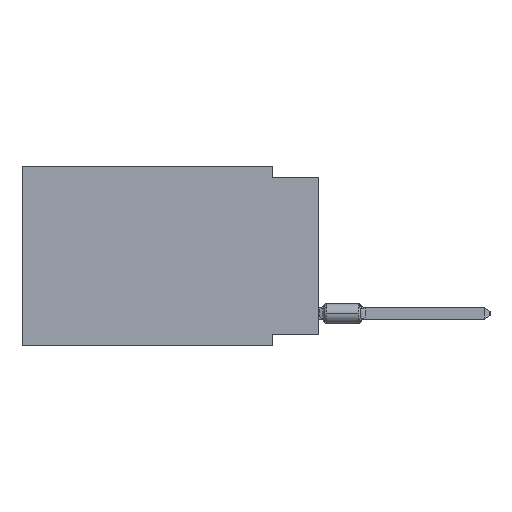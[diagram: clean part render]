
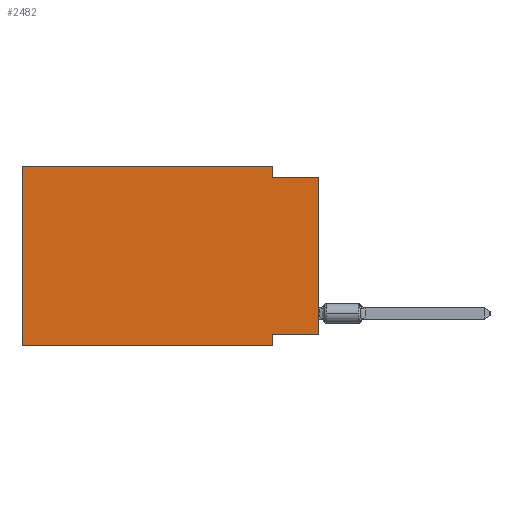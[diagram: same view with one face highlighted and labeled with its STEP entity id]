
A CAD part, left-side view. The second image highlights one B-rep face of the part: STEP entity #2482.
In plain terms, the highlighted planar face has unit normal (-1, 0, 0).
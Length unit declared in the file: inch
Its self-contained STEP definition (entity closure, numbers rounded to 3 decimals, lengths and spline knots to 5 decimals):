
#249 = CARTESIAN_POINT ( 'NONE',  ( 0., 0.645, -0.39 ) ) ;
#1726 = EDGE_LOOP ( 'NONE', ( #13828, #40966, #62145, #33426, #32283, #9849, #52335, #25994 ) ) ;
#2482 = ADVANCED_FACE ( 'NONE', ( #30068 ), #39983, .F. ) ;
#3877 = LINE ( 'NONE', #13837, #5460 ) ;
#5460 = VECTOR ( 'NONE', #45234, 39.37008 ) ;
#6135 = VECTOR ( 'NONE', #16411, 39.37008 ) ;
#6991 = CARTESIAN_POINT ( 'NONE',  ( 0., 0.645, 0. ) ) ;
#9849 = ORIENTED_EDGE ( 'NONE', *, *, #33218, .T. ) ;
#10283 = DIRECTION ( 'NONE',  ( 0., 1., 0. ) ) ;
#12593 = CARTESIAN_POINT ( 'NONE',  ( 0., 0., 0. ) ) ;
#13291 = CARTESIAN_POINT ( 'NONE',  ( 0., 0.645, -0.39 ) ) ;
#13553 = CARTESIAN_POINT ( 'NONE',  ( 0., 0.1, -0.39 ) ) ;
#13828 = ORIENTED_EDGE ( 'NONE', *, *, #42986, .T. ) ;
#13837 = CARTESIAN_POINT ( 'NONE',  ( 0., 0.1, -0.39 ) ) ;
#16411 = DIRECTION ( 'NONE',  ( 0., 0., -1. ) ) ;
#17756 = CARTESIAN_POINT ( 'NONE',  ( 0., 0., -0.025 ) ) ;
#19425 = EDGE_CURVE ( 'NONE', #52815, #37840, #35368, .T. ) ;
#21050 = VECTOR ( 'NONE', #21462, 39.37008 ) ;
#21462 = DIRECTION ( 'NONE',  ( 0., -1., 0. ) ) ;
#21525 = VECTOR ( 'NONE', #32927, 39.37008 ) ;
#21620 = DIRECTION ( 'NONE',  ( 0., -1., 0. ) ) ;
#24684 = LINE ( 'NONE', #249, #31939 ) ;
#25907 = EDGE_CURVE ( 'NONE', #57289, #54484, #37422, .T. ) ;
#25994 = ORIENTED_EDGE ( 'NONE', *, *, #40912, .F. ) ;
#26383 = CARTESIAN_POINT ( 'NONE',  ( 0., 0.1, 0. ) ) ;
#26460 = CARTESIAN_POINT ( 'NONE',  ( 0., 0.1, 0. ) ) ;
#28256 = VECTOR ( 'NONE', #32194, 39.37008 ) ;
#29109 = CARTESIAN_POINT ( 'NONE',  ( 0., 0., -0.025 ) ) ;
#30068 = FACE_OUTER_BOUND ( 'NONE', #1726, .T. ) ;
#30345 = EDGE_CURVE ( 'NONE', #47817, #35417, #3877, .T. ) ;
#30969 = CARTESIAN_POINT ( 'NONE',  ( 0., 0.1, -0.365 ) ) ;
#31939 = VECTOR ( 'NONE', #39721, 39.37008 ) ;
#32194 = DIRECTION ( 'NONE',  ( 0., 0., 1. ) ) ;
#32283 = ORIENTED_EDGE ( 'NONE', *, *, #25907, .F. ) ;
#32927 = DIRECTION ( 'NONE',  ( 0., 0., 1. ) ) ;
#33218 = EDGE_CURVE ( 'NONE', #57289, #35417, #24684, .T. ) ;
#33426 = ORIENTED_EDGE ( 'NONE', *, *, #44746, .F. ) ;
#35227 = EDGE_CURVE ( 'NONE', #37840, #43375, #51749, .T. ) ;
#35368 = LINE ( 'NONE', #26383, #6135 ) ;
#35417 = VERTEX_POINT ( 'NONE', #13553 ) ;
#37422 = LINE ( 'NONE', #47971, #21525 ) ;
#37595 = CARTESIAN_POINT ( 'NONE',  ( 0., 0.1, -0.025 ) ) ;
#37840 = VERTEX_POINT ( 'NONE', #37595 ) ;
#39190 = VERTEX_POINT ( 'NONE', #47925 ) ;
#39308 = VECTOR ( 'NONE', #21620, 39.37008 ) ;
#39668 = DIRECTION ( 'NONE',  ( 0., 0., -1. ) ) ;
#39721 = DIRECTION ( 'NONE',  ( 0., -1., 0. ) ) ;
#39983 = PLANE ( 'NONE',  #40197 ) ;
#40197 = AXIS2_PLACEMENT_3D ( 'NONE', #54104, #54422, #39668 ) ;
#40912 = EDGE_CURVE ( 'NONE', #39190, #47817, #59707, .T. ) ;
#40966 = ORIENTED_EDGE ( 'NONE', *, *, #35227, .F. ) ;
#42986 = EDGE_CURVE ( 'NONE', #39190, #43375, #56542, .T. ) ;
#43375 = VERTEX_POINT ( 'NONE', #29109 ) ;
#44746 = EDGE_CURVE ( 'NONE', #54484, #52815, #55132, .T. ) ;
#45234 = DIRECTION ( 'NONE',  ( 0., 0., -1. ) ) ;
#47817 = VERTEX_POINT ( 'NONE', #30969 ) ;
#47925 = CARTESIAN_POINT ( 'NONE',  ( 0., 0., -0.365 ) ) ;
#47971 = CARTESIAN_POINT ( 'NONE',  ( 0., 0.645, 0. ) ) ;
#51749 = LINE ( 'NONE', #17756, #39308 ) ;
#52335 = ORIENTED_EDGE ( 'NONE', *, *, #30345, .F. ) ;
#52815 = VERTEX_POINT ( 'NONE', #26460 ) ;
#54104 = CARTESIAN_POINT ( 'NONE',  ( 0., 0.645, 0. ) ) ;
#54422 = DIRECTION ( 'NONE',  ( 1., 0., 0. ) ) ;
#54484 = VERTEX_POINT ( 'NONE', #58166 ) ;
#54895 = CARTESIAN_POINT ( 'NONE',  ( 0., 0., -0.365 ) ) ;
#55132 = LINE ( 'NONE', #6991, #21050 ) ;
#56542 = LINE ( 'NONE', #12593, #28256 ) ;
#57289 = VERTEX_POINT ( 'NONE', #13291 ) ;
#58166 = CARTESIAN_POINT ( 'NONE',  ( 0., 0.645, 0. ) ) ;
#59707 = LINE ( 'NONE', #54895, #62849 ) ;
#62145 = ORIENTED_EDGE ( 'NONE', *, *, #19425, .F. ) ;
#62849 = VECTOR ( 'NONE', #10283, 39.37008 ) ;
